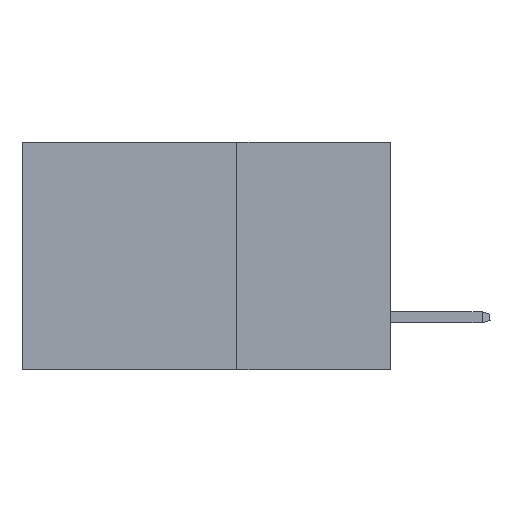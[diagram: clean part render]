
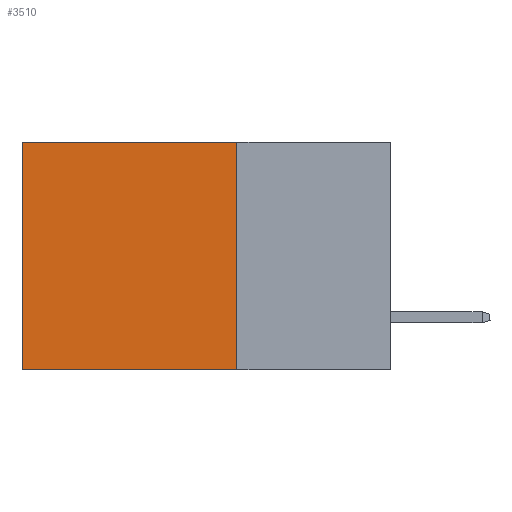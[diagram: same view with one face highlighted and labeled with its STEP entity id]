
A CAD part, left-side view. The second image highlights one B-rep face of the part: STEP entity #3510.
In plain terms, the highlighted planar face has unit normal (-1, 0, 0).
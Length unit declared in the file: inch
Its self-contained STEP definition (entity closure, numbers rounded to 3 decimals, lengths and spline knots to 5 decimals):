
#355 = LINE ( 'NONE', #18814, #11901 ) ;
#869 = CARTESIAN_POINT ( 'NONE',  ( 0.2875, 0.25, -0.37 ) ) ;
#1445 = VECTOR ( 'NONE', #4031, 39.37008 ) ;
#1650 = VECTOR ( 'NONE', #17845, 39.37008 ) ;
#1720 = ORIENTED_EDGE ( 'NONE', *, *, #14949, .T. ) ;
#2693 = CARTESIAN_POINT ( 'NONE',  ( 0.2875, 0.25, 0. ) ) ;
#3510 = ADVANCED_FACE ( 'NONE', ( #17470 ), #13092, .F. ) ;
#4031 = DIRECTION ( 'NONE',  ( 0., 0., -1. ) ) ;
#5148 = CARTESIAN_POINT ( 'NONE',  ( 0.2875, 0.6, 0. ) ) ;
#5937 = CARTESIAN_POINT ( 'NONE',  ( 0.2875, 0.6, -0.37 ) ) ;
#6115 = AXIS2_PLACEMENT_3D ( 'NONE', #9782, #16283, #8486 ) ;
#6158 = VECTOR ( 'NONE', #19593, 39.37008 ) ;
#6563 = CARTESIAN_POINT ( 'NONE',  ( 0.2875, 0.25, 0. ) ) ;
#7000 = CARTESIAN_POINT ( 'NONE',  ( 0.2875, 0.6, 0. ) ) ;
#8486 = DIRECTION ( 'NONE',  ( 0., 0., -1. ) ) ;
#8705 = ORIENTED_EDGE ( 'NONE', *, *, #15694, .F. ) ;
#8859 = CARTESIAN_POINT ( 'NONE',  ( 0.2875, 0.25, -0.37 ) ) ;
#9560 = DIRECTION ( 'NONE',  ( 0., 0., -1. ) ) ;
#9782 = CARTESIAN_POINT ( 'NONE',  ( 0.2875, 0.25, 0. ) ) ;
#10704 = VERTEX_POINT ( 'NONE', #5148 ) ;
#10755 = LINE ( 'NONE', #8859, #6158 ) ;
#10880 = VERTEX_POINT ( 'NONE', #6563 ) ;
#11454 = EDGE_CURVE ( 'NONE', #10880, #19570, #355, .T. ) ;
#11543 = LINE ( 'NONE', #7000, #1445 ) ;
#11901 = VECTOR ( 'NONE', #9560, 39.37008 ) ;
#12153 = VERTEX_POINT ( 'NONE', #5937 ) ;
#12482 = LINE ( 'NONE', #2693, #1650 ) ;
#13092 = PLANE ( 'NONE',  #6115 ) ;
#14949 = EDGE_CURVE ( 'NONE', #10880, #10704, #12482, .T. ) ;
#14973 = EDGE_LOOP ( 'NONE', ( #15855, #8705, #18356, #1720 ) ) ;
#15694 = EDGE_CURVE ( 'NONE', #19570, #12153, #10755, .T. ) ;
#15855 = ORIENTED_EDGE ( 'NONE', *, *, #18864, .T. ) ;
#16283 = DIRECTION ( 'NONE',  ( 1., 0., 0. ) ) ;
#17470 = FACE_OUTER_BOUND ( 'NONE', #14973, .T. ) ;
#17845 = DIRECTION ( 'NONE',  ( 0., 1., 0. ) ) ;
#18356 = ORIENTED_EDGE ( 'NONE', *, *, #11454, .F. ) ;
#18814 = CARTESIAN_POINT ( 'NONE',  ( 0.2875, 0.25, 0. ) ) ;
#18864 = EDGE_CURVE ( 'NONE', #10704, #12153, #11543, .T. ) ;
#19570 = VERTEX_POINT ( 'NONE', #869 ) ;
#19593 = DIRECTION ( 'NONE',  ( 0., 1., 0. ) ) ;
